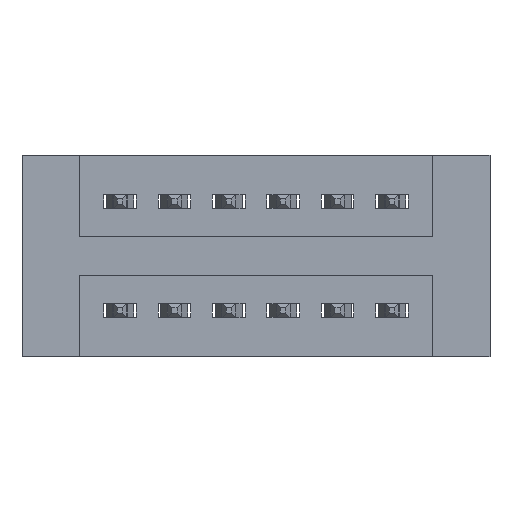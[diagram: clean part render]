
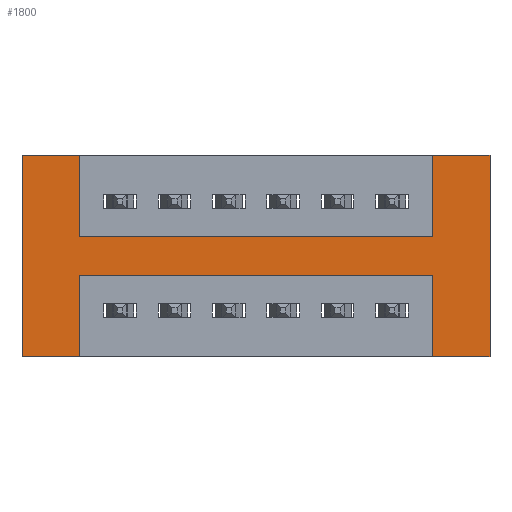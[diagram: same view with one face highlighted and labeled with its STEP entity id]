
A CAD part, front view. The second image highlights one B-rep face of the part: STEP entity #1800.
In plain terms, the highlighted planar face has unit normal (0, -1, 0).
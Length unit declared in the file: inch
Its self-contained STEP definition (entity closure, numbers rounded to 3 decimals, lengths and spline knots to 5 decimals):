
#47 = ORIENTED_EDGE ( 'NONE', *, *, #5517, .F. ) ;
#63 = ORIENTED_EDGE ( 'NONE', *, *, #297, .F. ) ;
#105 = DIRECTION ( 'NONE',  ( -1., 0., 0. ) ) ;
#114 = ORIENTED_EDGE ( 'NONE', *, *, #1487, .F. ) ;
#124 = ORIENTED_EDGE ( 'NONE', *, *, #9196, .F. ) ;
#155 = ORIENTED_EDGE ( 'NONE', *, *, #3036, .F. ) ;
#172 = ORIENTED_EDGE ( 'NONE', *, *, #8661, .F. ) ;
#275 = VERTEX_POINT ( 'NONE', #8887 ) ;
#297 = EDGE_CURVE ( 'NONE', #7434, #275, #2321, .T. ) ;
#359 = LINE ( 'NONE', #6831, #2077 ) ;
#527 = VERTEX_POINT ( 'NONE', #7538 ) ;
#560 = VECTOR ( 'NONE', #8697, 39.37008 ) ;
#648 = DIRECTION ( 'NONE',  ( 0., 0., 1. ) ) ;
#775 = EDGE_LOOP ( 'NONE', ( #3974, #63, #114, #124, #155, #172, #2249, #4464, #47, #4810, #7820, #2231 ) ) ;
#816 = VERTEX_POINT ( 'NONE', #4811 ) ;
#862 = VECTOR ( 'NONE', #7594, 39.37008 ) ;
#878 = CARTESIAN_POINT ( 'NONE',  ( 0.3925, 0., -0.22 ) ) ;
#989 = FACE_OUTER_BOUND ( 'NONE', #775, .T. ) ;
#1004 = VERTEX_POINT ( 'NONE', #4442 ) ;
#1212 = CARTESIAN_POINT ( 'NONE',  ( 1.0425, 0., 0. ) ) ;
#1248 = LINE ( 'NONE', #2190, #8782 ) ;
#1260 = AXIS2_PLACEMENT_3D ( 'NONE', #4226, #7117, #2114 ) ;
#1280 = DIRECTION ( 'NONE',  ( 1., 0., 0. ) ) ;
#1401 = CARTESIAN_POINT ( 'NONE',  ( 1.0425, 0., -0.15 ) ) ;
#1420 = VECTOR ( 'NONE', #1941, 39.37008 ) ;
#1432 = CARTESIAN_POINT ( 'NONE',  ( 0.2875, 0., 0. ) ) ;
#1487 = EDGE_CURVE ( 'NONE', #2560, #7434, #2397, .T. ) ;
#1699 = VERTEX_POINT ( 'NONE', #4352 ) ;
#1800 = ADVANCED_FACE ( 'NONE', ( #989 ), #8963, .T. ) ;
#1872 = VERTEX_POINT ( 'NONE', #8154 ) ;
#1941 = DIRECTION ( 'NONE',  ( 0., 0., -1. ) ) ;
#2015 = VECTOR ( 'NONE', #8454, 39.37008 ) ;
#2077 = VECTOR ( 'NONE', #3029, 39.37008 ) ;
#2114 = DIRECTION ( 'NONE',  ( 0., 0., -1. ) ) ;
#2190 = CARTESIAN_POINT ( 'NONE',  ( 1.1475, 0., 0. ) ) ;
#2231 = ORIENTED_EDGE ( 'NONE', *, *, #4667, .F. ) ;
#2249 = ORIENTED_EDGE ( 'NONE', *, *, #2546, .T. ) ;
#2308 = VERTEX_POINT ( 'NONE', #2471 ) ;
#2321 = LINE ( 'NONE', #8602, #7702 ) ;
#2397 = LINE ( 'NONE', #5055, #9310 ) ;
#2471 = CARTESIAN_POINT ( 'NONE',  ( 0.3925, 0., -0.15 ) ) ;
#2546 = EDGE_CURVE ( 'NONE', #4938, #816, #7087, .T. ) ;
#2560 = VERTEX_POINT ( 'NONE', #1401 ) ;
#2755 = CARTESIAN_POINT ( 'NONE',  ( 0.3925, 0., -0.37 ) ) ;
#2824 = VECTOR ( 'NONE', #5455, 39.37008 ) ;
#3029 = DIRECTION ( 'NONE',  ( 0., 0., 1. ) ) ;
#3036 = EDGE_CURVE ( 'NONE', #527, #2308, #9279, .T. ) ;
#3063 = VERTEX_POINT ( 'NONE', #3217 ) ;
#3217 = CARTESIAN_POINT ( 'NONE',  ( 0.3925, 0., -0.22 ) ) ;
#3486 = LINE ( 'NONE', #2755, #1420 ) ;
#3974 = ORIENTED_EDGE ( 'NONE', *, *, #8319, .T. ) ;
#4107 = CARTESIAN_POINT ( 'NONE',  ( 0.2875, 0., 0. ) ) ;
#4226 = CARTESIAN_POINT ( 'NONE',  ( 0., 0., -0.37 ) ) ;
#4352 = CARTESIAN_POINT ( 'NONE',  ( 1.0425, 0., -0.37 ) ) ;
#4442 = CARTESIAN_POINT ( 'NONE',  ( 0.3925, 0., -0.37 ) ) ;
#4464 = ORIENTED_EDGE ( 'NONE', *, *, #6609, .F. ) ;
#4534 = VECTOR ( 'NONE', #105, 39.37008 ) ;
#4613 = DIRECTION ( 'NONE',  ( 0., 0., -1. ) ) ;
#4667 = EDGE_CURVE ( 'NONE', #1872, #1699, #6430, .T. ) ;
#4688 = LINE ( 'NONE', #8026, #560 ) ;
#4810 = ORIENTED_EDGE ( 'NONE', *, *, #7876, .F. ) ;
#4811 = CARTESIAN_POINT ( 'NONE',  ( 0.2875, 0., -0.37 ) ) ;
#4830 = LINE ( 'NONE', #878, #2824 ) ;
#4938 = VERTEX_POINT ( 'NONE', #4107 ) ;
#5055 = CARTESIAN_POINT ( 'NONE',  ( 1.0425, 0., 0. ) ) ;
#5060 = CARTESIAN_POINT ( 'NONE',  ( 1.0425, 0., -0.22 ) ) ;
#5272 = DIRECTION ( 'NONE',  ( 0., 0., -1. ) ) ;
#5406 = CARTESIAN_POINT ( 'NONE',  ( 0.3925, 0., 0. ) ) ;
#5455 = DIRECTION ( 'NONE',  ( -1., 0., 0. ) ) ;
#5517 = EDGE_CURVE ( 'NONE', #3063, #1004, #3486, .T. ) ;
#5684 = EDGE_CURVE ( 'NONE', #1699, #6777, #359, .T. ) ;
#6335 = CARTESIAN_POINT ( 'NONE',  ( 0., 0., -0.37 ) ) ;
#6430 = LINE ( 'NONE', #7501, #4534 ) ;
#6609 = EDGE_CURVE ( 'NONE', #1004, #816, #6812, .T. ) ;
#6777 = VERTEX_POINT ( 'NONE', #5060 ) ;
#6812 = LINE ( 'NONE', #6335, #862 ) ;
#6831 = CARTESIAN_POINT ( 'NONE',  ( 1.0425, 0., -0.37 ) ) ;
#7087 = LINE ( 'NONE', #1432, #8374 ) ;
#7117 = DIRECTION ( 'NONE',  ( 0., -1., 0. ) ) ;
#7182 = DIRECTION ( 'NONE',  ( 0., 0., 1. ) ) ;
#7434 = VERTEX_POINT ( 'NONE', #1212 ) ;
#7501 = CARTESIAN_POINT ( 'NONE',  ( 0., 0., -0.37 ) ) ;
#7538 = CARTESIAN_POINT ( 'NONE',  ( 0.3925, 0., 0. ) ) ;
#7551 = VECTOR ( 'NONE', #5272, 39.37008 ) ;
#7594 = DIRECTION ( 'NONE',  ( -1., 0., 0. ) ) ;
#7632 = LINE ( 'NONE', #7778, #2015 ) ;
#7702 = VECTOR ( 'NONE', #1280, 39.37008 ) ;
#7778 = CARTESIAN_POINT ( 'NONE',  ( 0.3925, 0., -0.15 ) ) ;
#7820 = ORIENTED_EDGE ( 'NONE', *, *, #5684, .F. ) ;
#7876 = EDGE_CURVE ( 'NONE', #6777, #3063, #4830, .T. ) ;
#8026 = CARTESIAN_POINT ( 'NONE',  ( 0., 0., 0. ) ) ;
#8154 = CARTESIAN_POINT ( 'NONE',  ( 1.1475, 0., -0.37 ) ) ;
#8319 = EDGE_CURVE ( 'NONE', #1872, #275, #1248, .T. ) ;
#8374 = VECTOR ( 'NONE', #4613, 39.37008 ) ;
#8454 = DIRECTION ( 'NONE',  ( 1., 0., 0. ) ) ;
#8602 = CARTESIAN_POINT ( 'NONE',  ( 0., 0., 0. ) ) ;
#8661 = EDGE_CURVE ( 'NONE', #4938, #527, #4688, .T. ) ;
#8697 = DIRECTION ( 'NONE',  ( 1., 0., 0. ) ) ;
#8782 = VECTOR ( 'NONE', #7182, 39.37008 ) ;
#8887 = CARTESIAN_POINT ( 'NONE',  ( 1.1475, 0., 0. ) ) ;
#8963 = PLANE ( 'NONE',  #1260 ) ;
#9196 = EDGE_CURVE ( 'NONE', #2308, #2560, #7632, .T. ) ;
#9279 = LINE ( 'NONE', #5406, #7551 ) ;
#9310 = VECTOR ( 'NONE', #648, 39.37008 ) ;
